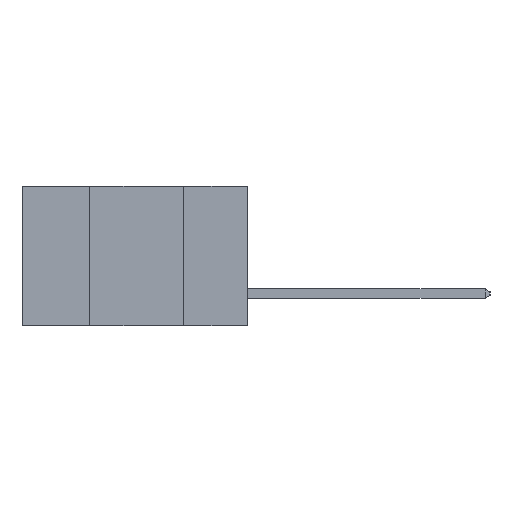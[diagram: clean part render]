
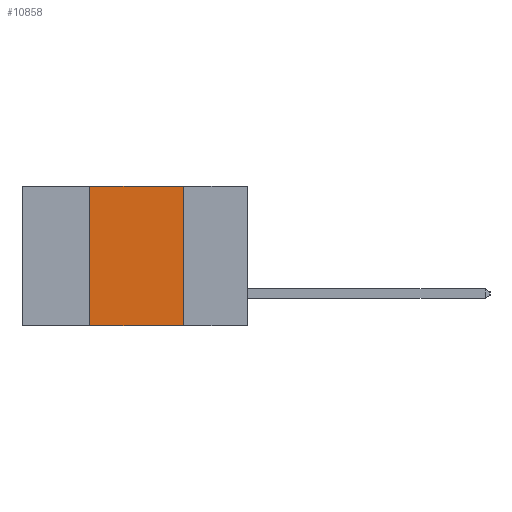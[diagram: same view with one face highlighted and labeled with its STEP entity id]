
A CAD part, left-side view. The second image highlights one B-rep face of the part: STEP entity #10858.
In plain terms, the highlighted planar face has unit normal (-1, 0, 0).
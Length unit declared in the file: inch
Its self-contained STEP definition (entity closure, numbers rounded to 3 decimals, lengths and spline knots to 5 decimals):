
#422 = LINE ( 'NONE', #4322, #1749 ) ;
#824 = EDGE_LOOP ( 'NONE', ( #9680, #8782, #20354, #10761 ) ) ;
#1002 = CARTESIAN_POINT ( 'NONE',  ( 0., 0.42, -0.37 ) ) ;
#1749 = VECTOR ( 'NONE', #4286, 39.37008 ) ;
#2060 = VECTOR ( 'NONE', #23861, 39.37008 ) ;
#2470 = LINE ( 'NONE', #1002, #18670 ) ;
#2701 = LINE ( 'NONE', #13919, #2060 ) ;
#3068 = DIRECTION ( 'NONE',  ( 0., 0., 1. ) ) ;
#3671 = DIRECTION ( 'NONE',  ( 0., 0., -1. ) ) ;
#3704 = DIRECTION ( 'NONE',  ( 1., 0., 0. ) ) ;
#3757 = CARTESIAN_POINT ( 'NONE',  ( 0., 0.6, 0. ) ) ;
#3798 = PLANE ( 'NONE',  #11612 ) ;
#4286 = DIRECTION ( 'NONE',  ( 0., -1., 0. ) ) ;
#4322 = CARTESIAN_POINT ( 'NONE',  ( 0., 0.6, 0. ) ) ;
#4646 = EDGE_CURVE ( 'NONE', #20526, #22488, #17975, .T. ) ;
#5155 = EDGE_CURVE ( 'NONE', #16052, #20526, #422, .T. ) ;
#8782 = ORIENTED_EDGE ( 'NONE', *, *, #5155, .F. ) ;
#9680 = ORIENTED_EDGE ( 'NONE', *, *, #4646, .F. ) ;
#10761 = ORIENTED_EDGE ( 'NONE', *, *, #14228, .T. ) ;
#10858 = ADVANCED_FACE ( 'NONE', ( #21236 ), #3798, .F. ) ;
#11612 = AXIS2_PLACEMENT_3D ( 'NONE', #3757, #3704, #3671 ) ;
#11786 = DIRECTION ( 'NONE',  ( 0., 0., -1. ) ) ;
#11865 = CARTESIAN_POINT ( 'NONE',  ( 0., 0.17, -0.37 ) ) ;
#12564 = VECTOR ( 'NONE', #11786, 39.37008 ) ;
#12587 = CARTESIAN_POINT ( 'NONE',  ( 0., 0.42, 0. ) ) ;
#13919 = CARTESIAN_POINT ( 'NONE',  ( 0., 0.6, -0.37 ) ) ;
#14228 = EDGE_CURVE ( 'NONE', #25664, #22488, #2701, .T. ) ;
#15088 = CARTESIAN_POINT ( 'NONE',  ( 0., 0.17, -0.37 ) ) ;
#16052 = VERTEX_POINT ( 'NONE', #12587 ) ;
#17975 = LINE ( 'NONE', #11865, #12564 ) ;
#18670 = VECTOR ( 'NONE', #3068, 39.37008 ) ;
#20354 = ORIENTED_EDGE ( 'NONE', *, *, #24938, .F. ) ;
#20526 = VERTEX_POINT ( 'NONE', #24540 ) ;
#21236 = FACE_OUTER_BOUND ( 'NONE', #824, .T. ) ;
#21670 = CARTESIAN_POINT ( 'NONE',  ( 0., 0.42, -0.37 ) ) ;
#22488 = VERTEX_POINT ( 'NONE', #15088 ) ;
#23861 = DIRECTION ( 'NONE',  ( 0., -1., 0. ) ) ;
#24540 = CARTESIAN_POINT ( 'NONE',  ( 0., 0.17, 0. ) ) ;
#24938 = EDGE_CURVE ( 'NONE', #25664, #16052, #2470, .T. ) ;
#25664 = VERTEX_POINT ( 'NONE', #21670 ) ;
